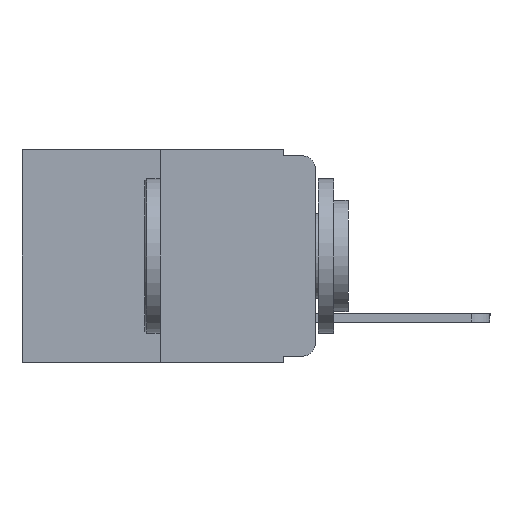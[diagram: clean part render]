
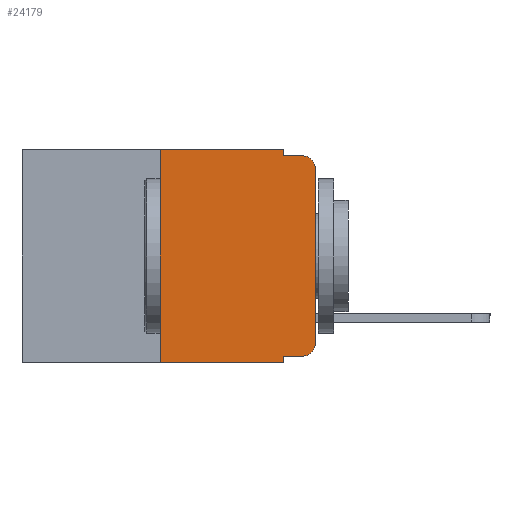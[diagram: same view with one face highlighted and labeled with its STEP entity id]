
A CAD part, left-side view. The second image highlights one B-rep face of the part: STEP entity #24179.
In plain terms, the highlighted planar face has unit normal (-1, 0, 0).
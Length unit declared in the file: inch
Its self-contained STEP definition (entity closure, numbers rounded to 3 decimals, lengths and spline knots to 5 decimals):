
#357 = ORIENTED_EDGE ( 'NONE', *, *, #20762, .F. ) ;
#476 = LINE ( 'NONE', #3770, #15919 ) ;
#508 = DIRECTION ( 'NONE',  ( 0., -1., 0. ) ) ;
#633 = DIRECTION ( 'NONE',  ( 0., -1., 0. ) ) ;
#939 = CARTESIAN_POINT ( 'NONE',  ( 0., 0.051, 0. ) ) ;
#941 = CARTESIAN_POINT ( 'NONE',  ( 0., 0.473, 0. ) ) ;
#1249 = ORIENTED_EDGE ( 'NONE', *, *, #11649, .T. ) ;
#1885 = EDGE_CURVE ( 'NONE', #19960, #4437, #18684, .T. ) ;
#2882 = CARTESIAN_POINT ( 'NONE',  ( 0., 0.473, 0. ) ) ;
#3062 = VERTEX_POINT ( 'NONE', #9635 ) ;
#3770 = CARTESIAN_POINT ( 'NONE',  ( 0., 0., 0. ) ) ;
#4028 = CARTESIAN_POINT ( 'NONE',  ( 0., 0.473, -0.343 ) ) ;
#4169 = VERTEX_POINT ( 'NONE', #12266 ) ;
#4437 = VERTEX_POINT ( 'NONE', #13953 ) ;
#4555 = DIRECTION ( 'NONE',  ( -1., 0., 0. ) ) ;
#4616 = ORIENTED_EDGE ( 'NONE', *, *, #13110, .F. ) ;
#4836 = EDGE_CURVE ( 'NONE', #19603, #15814, #24826, .T. ) ;
#5244 = VERTEX_POINT ( 'NONE', #20507 ) ;
#6135 = CARTESIAN_POINT ( 'NONE',  ( 0., 0.02, -0.333 ) ) ;
#7271 = DIRECTION ( 'NONE',  ( 0., 0., -1. ) ) ;
#7296 = EDGE_CURVE ( 'NONE', #4437, #5244, #476, .T. ) ;
#7380 = CARTESIAN_POINT ( 'NONE',  ( 0., 0.25, 0. ) ) ;
#7500 = VECTOR ( 'NONE', #20316, 39.37008 ) ;
#8051 = AXIS2_PLACEMENT_3D ( 'NONE', #19149, #21509, #21515 ) ;
#8883 = VECTOR ( 'NONE', #508, 39.37008 ) ;
#9061 = CARTESIAN_POINT ( 'NONE',  ( 0., 0.051, 0. ) ) ;
#9383 = VERTEX_POINT ( 'NONE', #10614 ) ;
#9415 = CARTESIAN_POINT ( 'NONE',  ( 0., 0.051, -0.01 ) ) ;
#9635 = CARTESIAN_POINT ( 'NONE',  ( 0., 0.25, 0. ) ) ;
#9939 = LINE ( 'NONE', #7380, #19609 ) ;
#10179 = CARTESIAN_POINT ( 'NONE',  ( 0., 0.051, -0.01 ) ) ;
#10354 = ORIENTED_EDGE ( 'NONE', *, *, #7296, .T. ) ;
#10614 = CARTESIAN_POINT ( 'NONE',  ( 0., 0.051, -0.333 ) ) ;
#10693 = DIRECTION ( 'NONE',  ( 1., 0., 0. ) ) ;
#11250 = DIRECTION ( 'NONE',  ( 0., 0., 1. ) ) ;
#11636 = AXIS2_PLACEMENT_3D ( 'NONE', #2882, #10693, #24242 ) ;
#11649 = EDGE_CURVE ( 'NONE', #5244, #18547, #13126, .T. ) ;
#12266 = CARTESIAN_POINT ( 'NONE',  ( 0., 0.051, -0.343 ) ) ;
#12479 = ORIENTED_EDGE ( 'NONE', *, *, #14376, .F. ) ;
#13110 = EDGE_CURVE ( 'NONE', #9383, #4169, #18453, .T. ) ;
#13126 = CIRCLE ( 'NONE', #20806, 0.02 ) ;
#13935 = VECTOR ( 'NONE', #7271, 39.37008 ) ;
#13953 = CARTESIAN_POINT ( 'NONE',  ( 0., 0., -0.313 ) ) ;
#14015 = LINE ( 'NONE', #10179, #8883 ) ;
#14376 = EDGE_CURVE ( 'NONE', #23281, #3062, #9939, .T. ) ;
#15360 = DIRECTION ( 'NONE',  ( 0., 0., 1. ) ) ;
#15814 = VERTEX_POINT ( 'NONE', #9415 ) ;
#15919 = VECTOR ( 'NONE', #15360, 39.37008 ) ;
#16108 = CARTESIAN_POINT ( 'NONE',  ( 0., 0.051, -0.333 ) ) ;
#16126 = CARTESIAN_POINT ( 'NONE',  ( 0., 0.02, -0.03 ) ) ;
#16478 = EDGE_CURVE ( 'NONE', #23281, #4169, #17368, .T. ) ;
#17290 = EDGE_CURVE ( 'NONE', #15814, #18547, #14015, .T. ) ;
#17368 = LINE ( 'NONE', #4028, #17968 ) ;
#17507 = CARTESIAN_POINT ( 'NONE',  ( 0., 0.02, -0.01 ) ) ;
#17681 = CARTESIAN_POINT ( 'NONE',  ( 0., 0.25, -0.343 ) ) ;
#17968 = VECTOR ( 'NONE', #21373, 39.37008 ) ;
#18053 = DIRECTION ( 'NONE',  ( 0., 0., -1. ) ) ;
#18453 = LINE ( 'NONE', #20786, #13935 ) ;
#18547 = VERTEX_POINT ( 'NONE', #17507 ) ;
#18684 = CIRCLE ( 'NONE', #8051, 0.02 ) ;
#19149 = CARTESIAN_POINT ( 'NONE',  ( 0., 0.02, -0.313 ) ) ;
#19471 = FACE_OUTER_BOUND ( 'NONE', #23813, .T. ) ;
#19603 = VERTEX_POINT ( 'NONE', #9061 ) ;
#19609 = VECTOR ( 'NONE', #11250, 39.37008 ) ;
#19960 = VERTEX_POINT ( 'NONE', #6135 ) ;
#20038 = EDGE_CURVE ( 'NONE', #9383, #19960, #20539, .T. ) ;
#20187 = DIRECTION ( 'NONE',  ( 0., 0., -1. ) ) ;
#20316 = DIRECTION ( 'NONE',  ( 0., -1., 0. ) ) ;
#20333 = PLANE ( 'NONE',  #11636 ) ;
#20507 = CARTESIAN_POINT ( 'NONE',  ( 0., 0., -0.03 ) ) ;
#20539 = LINE ( 'NONE', #16108, #25073 ) ;
#20762 = EDGE_CURVE ( 'NONE', #3062, #19603, #24134, .T. ) ;
#20786 = CARTESIAN_POINT ( 'NONE',  ( 0., 0.051, 0. ) ) ;
#20806 = AXIS2_PLACEMENT_3D ( 'NONE', #16126, #4555, #18053 ) ;
#21373 = DIRECTION ( 'NONE',  ( 0., -1., 0. ) ) ;
#21509 = DIRECTION ( 'NONE',  ( -1., 0., 0. ) ) ;
#21515 = DIRECTION ( 'NONE',  ( 0., 0., -1. ) ) ;
#22385 = VECTOR ( 'NONE', #20187, 39.37008 ) ;
#22490 = ORIENTED_EDGE ( 'NONE', *, *, #20038, .T. ) ;
#23075 = ORIENTED_EDGE ( 'NONE', *, *, #17290, .F. ) ;
#23096 = ORIENTED_EDGE ( 'NONE', *, *, #1885, .T. ) ;
#23281 = VERTEX_POINT ( 'NONE', #17681 ) ;
#23813 = EDGE_LOOP ( 'NONE', ( #10354, #1249, #23075, #24896, #357, #12479, #23992, #4616, #22490, #23096 ) ) ;
#23992 = ORIENTED_EDGE ( 'NONE', *, *, #16478, .T. ) ;
#24134 = LINE ( 'NONE', #941, #7500 ) ;
#24179 = ADVANCED_FACE ( 'NONE', ( #19471 ), #20333, .F. ) ;
#24242 = DIRECTION ( 'NONE',  ( 0., 0., -1. ) ) ;
#24826 = LINE ( 'NONE', #939, #22385 ) ;
#24896 = ORIENTED_EDGE ( 'NONE', *, *, #4836, .F. ) ;
#25073 = VECTOR ( 'NONE', #633, 39.37008 ) ;
